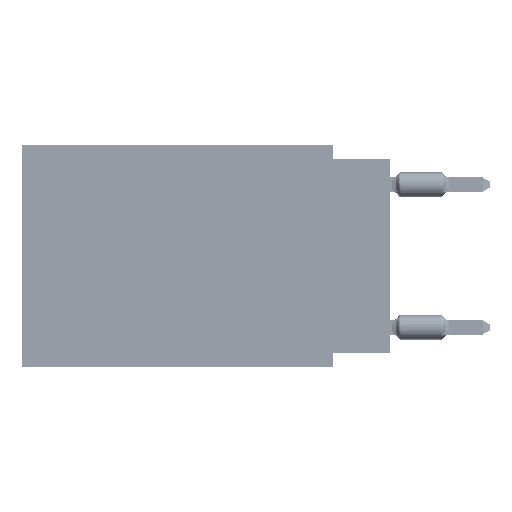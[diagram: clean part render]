
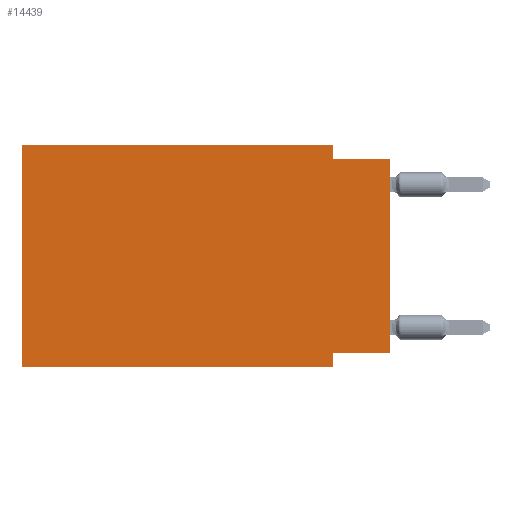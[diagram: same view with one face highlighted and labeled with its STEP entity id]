
A CAD part, left-side view. The second image highlights one B-rep face of the part: STEP entity #14439.
In plain terms, the highlighted planar face has unit normal (-1, 0, 0).
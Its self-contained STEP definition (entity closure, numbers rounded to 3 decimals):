
#2540 = ORIENTED_EDGE ( 'NONE', *, *, #56332, .F. ) ;
#2655 = ORIENTED_EDGE ( 'NONE', *, *, #2918, .T. ) ;
#2918 = EDGE_CURVE ( 'NONE', #56866, #49536, #24044, .T. ) ;
#2932 = ORIENTED_EDGE ( 'NONE', *, *, #3667, .F. ) ;
#3094 = PLANE ( 'NONE',  #56686 ) ;
#3161 = VECTOR ( 'NONE', #24817, 1000. ) ;
#3667 = EDGE_CURVE ( 'NONE', #8618, #35404, #19875, .T. ) ;
#3875 = LINE ( 'NONE', #13417, #17152 ) ;
#7882 = LINE ( 'NONE', #59562, #49471 ) ;
#8493 = DIRECTION ( 'NONE',  ( 0., 0., -1. ) ) ;
#8618 = VERTEX_POINT ( 'NONE', #38107 ) ;
#9316 = VECTOR ( 'NONE', #36751, 1000. ) ;
#9335 = VECTOR ( 'NONE', #19745, 1000. ) ;
#10353 = CARTESIAN_POINT ( 'NONE',  ( 0., 2.54, 0. ) ) ;
#10374 = ORIENTED_EDGE ( 'NONE', *, *, #26601, .F. ) ;
#11171 = CARTESIAN_POINT ( 'NONE',  ( 0., 2.54, -9.906 ) ) ;
#12311 = DIRECTION ( 'NONE',  ( 1., 0., 0. ) ) ;
#12512 = ORIENTED_EDGE ( 'NONE', *, *, #17488, .F. ) ;
#12801 = CARTESIAN_POINT ( 'NONE',  ( 0., 0., -0.635 ) ) ;
#13417 = CARTESIAN_POINT ( 'NONE',  ( 0., 2.54, -9.906 ) ) ;
#14439 = ADVANCED_FACE ( 'NONE', ( #40604 ), #3094, .F. ) ;
#15885 = VECTOR ( 'NONE', #19417, 1000. ) ;
#17152 = VECTOR ( 'NONE', #8493, 1000. ) ;
#17488 = EDGE_CURVE ( 'NONE', #52936, #8618, #51668, .T. ) ;
#17848 = DIRECTION ( 'NONE',  ( 0., -1., 0. ) ) ;
#17986 = LINE ( 'NONE', #12801, #9316 ) ;
#18549 = CARTESIAN_POINT ( 'NONE',  ( 0., 0., -0.635 ) ) ;
#19417 = DIRECTION ( 'NONE',  ( 0., 0., 1. ) ) ;
#19745 = DIRECTION ( 'NONE',  ( 0., 1., 0. ) ) ;
#19875 = LINE ( 'NONE', #10353, #3161 ) ;
#20354 = LINE ( 'NONE', #38212, #9335 ) ;
#23109 = ORIENTED_EDGE ( 'NONE', *, *, #56186, .T. ) ;
#24044 = LINE ( 'NONE', #42800, #15885 ) ;
#24817 = DIRECTION ( 'NONE',  ( 0., 0., -1. ) ) ;
#26601 = EDGE_CURVE ( 'NONE', #56866, #32083, #20354, .T. ) ;
#28539 = CARTESIAN_POINT ( 'NONE',  ( 0., 2.54, -0.635 ) ) ;
#29266 = ORIENTED_EDGE ( 'NONE', *, *, #39472, .F. ) ;
#32083 = VERTEX_POINT ( 'NONE', #52601 ) ;
#32202 = ORIENTED_EDGE ( 'NONE', *, *, #38327, .F. ) ;
#34472 = CARTESIAN_POINT ( 'NONE',  ( 0., 16.383, -9.906 ) ) ;
#35109 = VECTOR ( 'NONE', #17848, 1000. ) ;
#35404 = VERTEX_POINT ( 'NONE', #28539 ) ;
#35559 = DIRECTION ( 'NONE',  ( 0., -1., 0. ) ) ;
#36173 = DIRECTION ( 'NONE',  ( 0., 0., 1. ) ) ;
#36751 = DIRECTION ( 'NONE',  ( 0., -1., 0. ) ) ;
#38107 = CARTESIAN_POINT ( 'NONE',  ( 0., 2.54, 0. ) ) ;
#38192 = CARTESIAN_POINT ( 'NONE',  ( 0., 0., -9.271 ) ) ;
#38212 = CARTESIAN_POINT ( 'NONE',  ( 0., 0., -9.271 ) ) ;
#38327 = EDGE_CURVE ( 'NONE', #53920, #52936, #7882, .T. ) ;
#39472 = EDGE_CURVE ( 'NONE', #32083, #59423, #3875, .T. ) ;
#39980 = CARTESIAN_POINT ( 'NONE',  ( 0., 16.383, 0. ) ) ;
#40604 = FACE_OUTER_BOUND ( 'NONE', #52327, .T. ) ;
#42800 = CARTESIAN_POINT ( 'NONE',  ( 0., 0., 0. ) ) ;
#45235 = CARTESIAN_POINT ( 'NONE',  ( 0., 16.383, 0. ) ) ;
#48640 = VECTOR ( 'NONE', #35559, 1000. ) ;
#49471 = VECTOR ( 'NONE', #36173, 1000. ) ;
#49536 = VERTEX_POINT ( 'NONE', #18549 ) ;
#50155 = DIRECTION ( 'NONE',  ( 0., 0., -1. ) ) ;
#51072 = CARTESIAN_POINT ( 'NONE',  ( 0., 16.383, 0. ) ) ;
#51668 = LINE ( 'NONE', #51072, #35109 ) ;
#52327 = EDGE_LOOP ( 'NONE', ( #2655, #2540, #2932, #12512, #32202, #23109, #29266, #10374 ) ) ;
#52601 = CARTESIAN_POINT ( 'NONE',  ( 0., 2.54, -9.271 ) ) ;
#52936 = VERTEX_POINT ( 'NONE', #39980 ) ;
#53920 = VERTEX_POINT ( 'NONE', #34472 ) ;
#54025 = CARTESIAN_POINT ( 'NONE',  ( 0., 16.383, -9.906 ) ) ;
#56186 = EDGE_CURVE ( 'NONE', #53920, #59423, #58033, .T. ) ;
#56332 = EDGE_CURVE ( 'NONE', #35404, #49536, #17986, .T. ) ;
#56686 = AXIS2_PLACEMENT_3D ( 'NONE', #45235, #12311, #50155 ) ;
#56866 = VERTEX_POINT ( 'NONE', #38192 ) ;
#58033 = LINE ( 'NONE', #54025, #48640 ) ;
#59423 = VERTEX_POINT ( 'NONE', #11171 ) ;
#59562 = CARTESIAN_POINT ( 'NONE',  ( 0., 16.383, 0. ) ) ;
